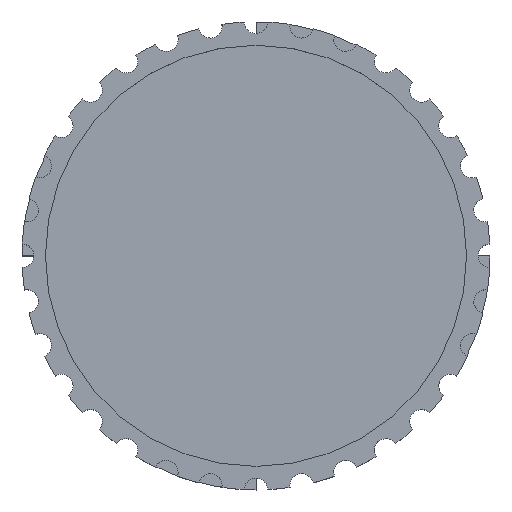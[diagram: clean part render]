
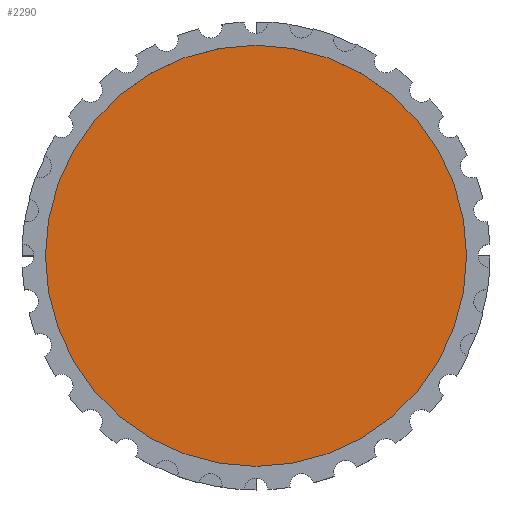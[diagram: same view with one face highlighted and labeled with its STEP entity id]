
A CAD part, top view. The second image highlights one B-rep face of the part: STEP entity #2290.
In plain terms, the highlighted planar face has unit normal (0, 0, 1).
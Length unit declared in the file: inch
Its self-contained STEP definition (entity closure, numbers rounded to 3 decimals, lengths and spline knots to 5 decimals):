
#119 = EDGE_LOOP ( 'NONE', ( #2428, #990 ) ) ;
#472 = DIRECTION ( 'NONE',  ( 1., 0., 0. ) ) ;
#639 = CARTESIAN_POINT ( 'NONE',  ( 0., 0., 0.26063 ) ) ;
#647 = CIRCLE ( 'NONE', #3114, 0.5625 ) ;
#933 = DIRECTION ( 'NONE',  ( 0., 0., 1. ) ) ;
#942 = CARTESIAN_POINT ( 'NONE',  ( -0.5625, 0., 0.26063 ) ) ;
#990 = ORIENTED_EDGE ( 'NONE', *, *, #1473, .T. ) ;
#1051 = CARTESIAN_POINT ( 'NONE',  ( 0., 0., 0.26063 ) ) ;
#1473 = EDGE_CURVE ( 'NONE', #2060, #2557, #2922, .T. ) ;
#2060 = VERTEX_POINT ( 'NONE', #942 ) ;
#2143 = DIRECTION ( 'NONE',  ( 1., 0., 0. ) ) ;
#2290 = ADVANCED_FACE ( 'NONE', ( #2478 ), #2710, .T. ) ;
#2428 = ORIENTED_EDGE ( 'NONE', *, *, #3211, .T. ) ;
#2468 = AXIS2_PLACEMENT_3D ( 'NONE', #1051, #3743, #2143 ) ;
#2478 = FACE_OUTER_BOUND ( 'NONE', #119, .T. ) ;
#2557 = VERTEX_POINT ( 'NONE', #2855 ) ;
#2664 = CARTESIAN_POINT ( 'NONE',  ( 0., 0., 0.26063 ) ) ;
#2710 = PLANE ( 'NONE',  #3214 ) ;
#2855 = CARTESIAN_POINT ( 'NONE',  ( 0.5625, 0., 0.26063 ) ) ;
#2922 = CIRCLE ( 'NONE', #2468, 0.5625 ) ;
#2993 = DIRECTION ( 'NONE',  ( 0., 0., 1. ) ) ;
#3114 = AXIS2_PLACEMENT_3D ( 'NONE', #639, #933, #3523 ) ;
#3211 = EDGE_CURVE ( 'NONE', #2557, #2060, #647, .T. ) ;
#3214 = AXIS2_PLACEMENT_3D ( 'NONE', #2664, #2993, #472 ) ;
#3523 = DIRECTION ( 'NONE',  ( 1., 0., 0. ) ) ;
#3743 = DIRECTION ( 'NONE',  ( 0., 0., 1. ) ) ;
